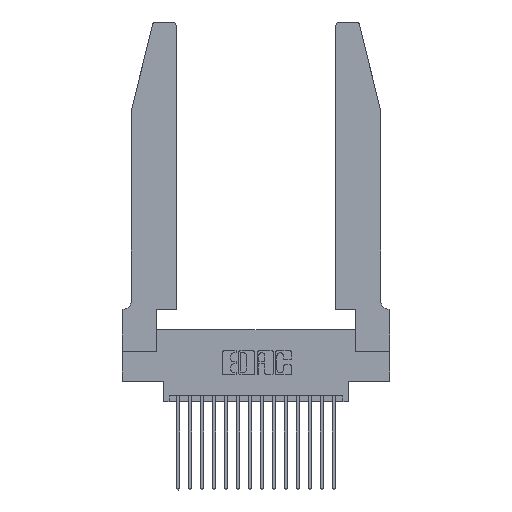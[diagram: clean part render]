
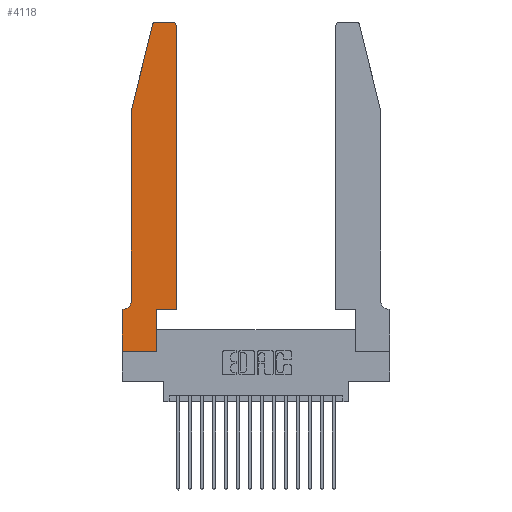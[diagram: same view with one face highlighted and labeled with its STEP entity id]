
A CAD part, top view. The second image highlights one B-rep face of the part: STEP entity #4118.
In plain terms, the highlighted planar face has unit normal (0, 0, 1).
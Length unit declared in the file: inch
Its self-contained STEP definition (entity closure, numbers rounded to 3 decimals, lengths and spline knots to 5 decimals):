
#30 = VERTEX_POINT ( 'NONE', #10282 ) ;
#51 = VERTEX_POINT ( 'NONE', #9203 ) ;
#540 = VECTOR ( 'NONE', #1335, 39.37008 ) ;
#698 = LINE ( 'NONE', #15505, #8291 ) ;
#933 = CARTESIAN_POINT ( 'NONE',  ( 0.0755, 0.42, 0.37 ) ) ;
#1180 = VECTOR ( 'NONE', #4697, 39.37008 ) ;
#1335 = DIRECTION ( 'NONE',  ( 1., 0., 0. ) ) ;
#2906 = ORIENTED_EDGE ( 'NONE', *, *, #16863, .T. ) ;
#3006 = LINE ( 'NONE', #18531, #3486 ) ;
#3037 = CARTESIAN_POINT ( 'NONE',  ( 0., 0.35, 0.37 ) ) ;
#3068 = FACE_OUTER_BOUND ( 'NONE', #5153, .T. ) ;
#3126 = DIRECTION ( 'NONE',  ( 0., 1., 0. ) ) ;
#3328 = CARTESIAN_POINT ( 'NONE',  ( 0.2865, 0.35, 0.37 ) ) ;
#3486 = VECTOR ( 'NONE', #12230, 39.37008 ) ;
#3643 = CARTESIAN_POINT ( 'NONE',  ( 0.0055, 0.42, 0.37 ) ) ;
#3745 = AXIS2_PLACEMENT_3D ( 'NONE', #3643, #3838, #17548 ) ;
#3838 = DIRECTION ( 'NONE',  ( 0., 0., -1. ) ) ;
#4118 = ADVANCED_FACE ( 'NONE', ( #3068 ), #13583, .T. ) ;
#4250 = VECTOR ( 'NONE', #10439, 39.37008 ) ;
#4430 = CARTESIAN_POINT ( 'NONE',  ( 0.0755, 2., 0.37 ) ) ;
#4482 = DIRECTION ( 'NONE',  ( 0., 0., 1. ) ) ;
#4577 = VECTOR ( 'NONE', #8874, 39.37008 ) ;
#4657 = DIRECTION ( 'NONE',  ( 1., 0., 0. ) ) ;
#4697 = DIRECTION ( 'NONE',  ( 0., -1., 0. ) ) ;
#4736 = ORIENTED_EDGE ( 'NONE', *, *, #18473, .T. ) ;
#5153 = EDGE_LOOP ( 'NONE', ( #5960, #16463, #17820, #4736, #8681, #12588, #6510, #2906, #9646, #10468, #7191, #12351 ) ) ;
#5181 = VERTEX_POINT ( 'NONE', #7556 ) ;
#5640 = LINE ( 'NONE', #15203, #10387 ) ;
#5716 = VERTEX_POINT ( 'NONE', #10447 ) ;
#5727 = EDGE_CURVE ( 'NONE', #15099, #17942, #5640, .T. ) ;
#5740 = DIRECTION ( 'NONE',  ( 1., 0., 0. ) ) ;
#5826 = CIRCLE ( 'NONE', #3745, 0.07 ) ;
#5859 = CARTESIAN_POINT ( 'NONE',  ( 0.0755, 0.35, 0.37 ) ) ;
#5960 = ORIENTED_EDGE ( 'NONE', *, *, #6715, .T. ) ;
#6020 = CARTESIAN_POINT ( 'NONE',  ( 0.2865, 0., 0.37 ) ) ;
#6158 = LINE ( 'NONE', #11936, #4250 ) ;
#6510 = ORIENTED_EDGE ( 'NONE', *, *, #6592, .T. ) ;
#6592 = EDGE_CURVE ( 'NONE', #14292, #12034, #18496, .T. ) ;
#6715 = EDGE_CURVE ( 'NONE', #30, #5181, #3006, .T. ) ;
#7076 = EDGE_CURVE ( 'NONE', #5181, #13291, #13655, .T. ) ;
#7191 = ORIENTED_EDGE ( 'NONE', *, *, #16302, .T. ) ;
#7423 = LINE ( 'NONE', #5859, #4577 ) ;
#7426 = CARTESIAN_POINT ( 'NONE',  ( 0., 0., 0.37 ) ) ;
#7556 = CARTESIAN_POINT ( 'NONE',  ( 0.284, 2.75, 0.37 ) ) ;
#7699 = EDGE_CURVE ( 'NONE', #18899, #14541, #5826, .T. ) ;
#8291 = VECTOR ( 'NONE', #4657, 39.37008 ) ;
#8681 = ORIENTED_EDGE ( 'NONE', *, *, #7699, .T. ) ;
#8737 = CARTESIAN_POINT ( 'NONE',  ( 0.284, 2.72, 0.37 ) ) ;
#8874 = DIRECTION ( 'NONE',  ( -1., 0., 0. ) ) ;
#8956 = DIRECTION ( 'NONE',  ( 0., -1., 0. ) ) ;
#9006 = CARTESIAN_POINT ( 'NONE',  ( 0., 0., 0.37 ) ) ;
#9203 = CARTESIAN_POINT ( 'NONE',  ( 0.0755, 2., 0.37 ) ) ;
#9476 = AXIS2_PLACEMENT_3D ( 'NONE', #18388, #18586, #12498 ) ;
#9646 = ORIENTED_EDGE ( 'NONE', *, *, #5727, .T. ) ;
#9782 = LINE ( 'NONE', #4430, #16677 ) ;
#9786 = CIRCLE ( 'NONE', #9476, 0.03 ) ;
#10282 = CARTESIAN_POINT ( 'NONE',  ( 0.4205, 2.75, 0.37 ) ) ;
#10387 = VECTOR ( 'NONE', #3126, 39.37008 ) ;
#10439 = DIRECTION ( 'NONE',  ( 0., 1., 0. ) ) ;
#10447 = CARTESIAN_POINT ( 'NONE',  ( 0.4505, 2.72, 0.37 ) ) ;
#10458 = CARTESIAN_POINT ( 'NONE',  ( 0., 0., 0.37 ) ) ;
#10468 = ORIENTED_EDGE ( 'NONE', *, *, #14141, .T. ) ;
#10751 = CARTESIAN_POINT ( 'NONE',  ( 0.0055, 0.35, 0.37 ) ) ;
#10817 = CARTESIAN_POINT ( 'NONE',  ( 0.4505, 0.35, 0.37 ) ) ;
#11690 = LINE ( 'NONE', #7426, #540 ) ;
#11936 = CARTESIAN_POINT ( 'NONE',  ( 0.4505, 0.35, 0.37 ) ) ;
#12034 = VERTEX_POINT ( 'NONE', #10458 ) ;
#12230 = DIRECTION ( 'NONE',  ( -1., 0., 0. ) ) ;
#12316 = CARTESIAN_POINT ( 'NONE',  ( 0.0755, 2., 0.37 ) ) ;
#12351 = ORIENTED_EDGE ( 'NONE', *, *, #15845, .T. ) ;
#12498 = DIRECTION ( 'NONE',  ( 1., 0., 0. ) ) ;
#12588 = ORIENTED_EDGE ( 'NONE', *, *, #13669, .T. ) ;
#13291 = VERTEX_POINT ( 'NONE', #15603 ) ;
#13578 = DIRECTION ( 'NONE',  ( -0.239, -0.971, 0. ) ) ;
#13583 = PLANE ( 'NONE',  #18758 ) ;
#13655 = CIRCLE ( 'NONE', #16111, 0.03 ) ;
#13669 = EDGE_CURVE ( 'NONE', #14541, #14292, #7423, .T. ) ;
#14141 = EDGE_CURVE ( 'NONE', #17942, #18489, #698, .T. ) ;
#14292 = VERTEX_POINT ( 'NONE', #17455 ) ;
#14541 = VERTEX_POINT ( 'NONE', #10751 ) ;
#15063 = EDGE_CURVE ( 'NONE', #13291, #51, #9782, .T. ) ;
#15099 = VERTEX_POINT ( 'NONE', #6020 ) ;
#15187 = LINE ( 'NONE', #12316, #1180 ) ;
#15203 = CARTESIAN_POINT ( 'NONE',  ( 0.2865, 0.35, 0.37 ) ) ;
#15505 = CARTESIAN_POINT ( 'NONE',  ( 0.4505, 0.35, 0.37 ) ) ;
#15603 = CARTESIAN_POINT ( 'NONE',  ( 0.25487, 2.72718, 0.37 ) ) ;
#15845 = EDGE_CURVE ( 'NONE', #5716, #30, #9786, .T. ) ;
#16111 = AXIS2_PLACEMENT_3D ( 'NONE', #8737, #16315, #5740 ) ;
#16302 = EDGE_CURVE ( 'NONE', #18489, #5716, #6158, .T. ) ;
#16315 = DIRECTION ( 'NONE',  ( 0., 0., 1. ) ) ;
#16463 = ORIENTED_EDGE ( 'NONE', *, *, #7076, .T. ) ;
#16656 = DIRECTION ( 'NONE',  ( 1., 0., 0. ) ) ;
#16677 = VECTOR ( 'NONE', #13578, 39.37008 ) ;
#16863 = EDGE_CURVE ( 'NONE', #12034, #15099, #11690, .T. ) ;
#17455 = CARTESIAN_POINT ( 'NONE',  ( 0., 0.35, 0.37 ) ) ;
#17534 = VECTOR ( 'NONE', #8956, 39.37008 ) ;
#17548 = DIRECTION ( 'NONE',  ( -1., 0., 0. ) ) ;
#17820 = ORIENTED_EDGE ( 'NONE', *, *, #15063, .T. ) ;
#17942 = VERTEX_POINT ( 'NONE', #3328 ) ;
#18388 = CARTESIAN_POINT ( 'NONE',  ( 0.4205, 2.72, 0.37 ) ) ;
#18473 = EDGE_CURVE ( 'NONE', #51, #18899, #15187, .T. ) ;
#18489 = VERTEX_POINT ( 'NONE', #10817 ) ;
#18496 = LINE ( 'NONE', #9006, #17534 ) ;
#18531 = CARTESIAN_POINT ( 'NONE',  ( 0.2605, 2.75, 0.37 ) ) ;
#18586 = DIRECTION ( 'NONE',  ( 0., 0., 1. ) ) ;
#18758 = AXIS2_PLACEMENT_3D ( 'NONE', #3037, #4482, #16656 ) ;
#18899 = VERTEX_POINT ( 'NONE', #933 ) ;
